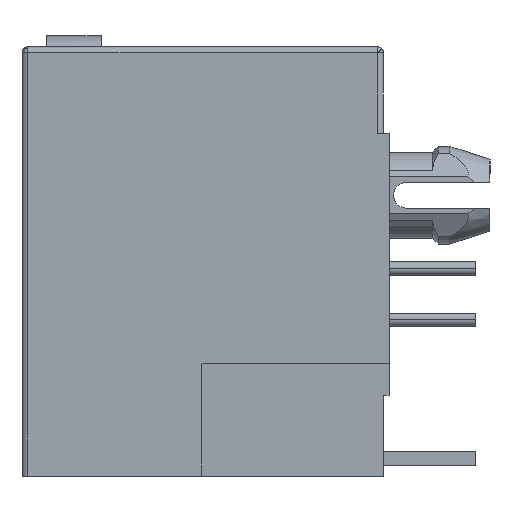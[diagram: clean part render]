
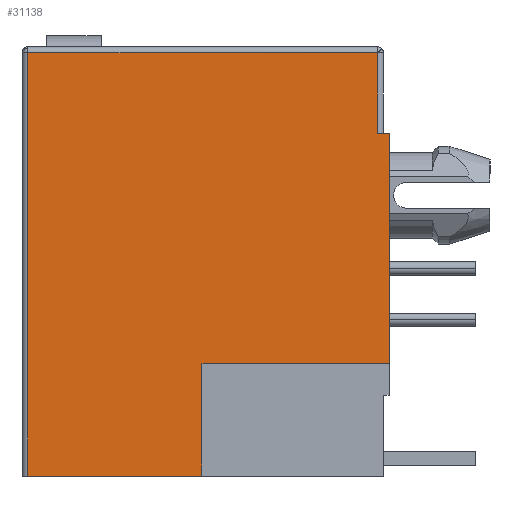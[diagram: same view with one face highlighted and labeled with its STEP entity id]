
A CAD part, left-side view. The second image highlights one B-rep face of the part: STEP entity #31138.
In plain terms, the highlighted planar face has unit normal (-1, 0, 0).
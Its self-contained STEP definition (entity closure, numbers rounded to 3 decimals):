
#608 = AXIS2_PLACEMENT_3D ( 'NONE', #10831, #44853, #58701 ) ;
#704 = CARTESIAN_POINT ( 'NONE',  ( -8.025, -0.125, -3.475 ) ) ;
#1014 = DIRECTION ( 'NONE',  ( 0., 0., 1. ) ) ;
#3329 = VECTOR ( 'NONE', #15140, 1000. ) ;
#4079 = LINE ( 'NONE', #29291, #36528 ) ;
#4708 = EDGE_CURVE ( 'NONE', #26105, #23513, #4079, .T. ) ;
#5362 = EDGE_CURVE ( 'NONE', #15642, #38719, #58306, .T. ) ;
#6454 = CARTESIAN_POINT ( 'NONE',  ( -8.025, 0., -7.375 ) ) ;
#9864 = CARTESIAN_POINT ( 'NONE',  ( -8.025, -6.225, 4.525 ) ) ;
#9989 = VECTOR ( 'NONE', #34020, 1000. ) ;
#10191 = EDGE_LOOP ( 'NONE', ( #31812, #27257, #27498, #35029, #23617, #24989, #46596, #56977 ) ) ;
#10323 = CARTESIAN_POINT ( 'NONE',  ( -8.025, 5.925, 26.949 ) ) ;
#10831 = CARTESIAN_POINT ( 'NONE',  ( -8.025, 0., 0. ) ) ;
#11187 = EDGE_CURVE ( 'NONE', #23513, #20671, #41439, .T. ) ;
#12280 = VERTEX_POINT ( 'NONE', #40879 ) ;
#13189 = CARTESIAN_POINT ( 'NONE',  ( -8.025, -6.625, 4.525 ) ) ;
#15140 = DIRECTION ( 'NONE',  ( 0., -1., 0. ) ) ;
#15278 = PLANE ( 'NONE',  #608 ) ;
#15302 = CARTESIAN_POINT ( 'NONE',  ( -8.025, 0., -3.475 ) ) ;
#15557 = VERTEX_POINT ( 'NONE', #38076 ) ;
#15642 = VERTEX_POINT ( 'NONE', #704 ) ;
#20671 = VERTEX_POINT ( 'NONE', #45750 ) ;
#20880 = VECTOR ( 'NONE', #41548, 1000. ) ;
#22451 = CARTESIAN_POINT ( 'NONE',  ( -8.025, 0., 7.325 ) ) ;
#23513 = VERTEX_POINT ( 'NONE', #59737 ) ;
#23617 = ORIENTED_EDGE ( 'NONE', *, *, #4708, .T. ) ;
#24989 = ORIENTED_EDGE ( 'NONE', *, *, #11187, .T. ) ;
#25247 = LINE ( 'NONE', #6454, #3329 ) ;
#25797 = EDGE_CURVE ( 'NONE', #38719, #28147, #35247, .T. ) ;
#26105 = VERTEX_POINT ( 'NONE', #9864 ) ;
#26622 = FACE_OUTER_BOUND ( 'NONE', #10191, .T. ) ;
#27257 = ORIENTED_EDGE ( 'NONE', *, *, #5362, .T. ) ;
#27498 = ORIENTED_EDGE ( 'NONE', *, *, #25797, .T. ) ;
#28147 = VERTEX_POINT ( 'NONE', #13189 ) ;
#29291 = CARTESIAN_POINT ( 'NONE',  ( -8.025, -6.225, 0. ) ) ;
#29880 = VECTOR ( 'NONE', #36576, 1000. ) ;
#31138 = ADVANCED_FACE ( 'NONE', ( #26622 ), #15278, .T. ) ;
#31812 = ORIENTED_EDGE ( 'NONE', *, *, #43399, .T. ) ;
#32151 = DIRECTION ( 'NONE',  ( 0., 1., 0. ) ) ;
#33746 = DIRECTION ( 'NONE',  ( 0., 0., 1. ) ) ;
#34020 = DIRECTION ( 'NONE',  ( 0., 1., 0. ) ) ;
#35029 = ORIENTED_EDGE ( 'NONE', *, *, #61940, .T. ) ;
#35247 = LINE ( 'NONE', #37299, #20880 ) ;
#36528 = VECTOR ( 'NONE', #1014, 1000. ) ;
#36576 = DIRECTION ( 'NONE',  ( 0., 0., 1. ) ) ;
#37299 = CARTESIAN_POINT ( 'NONE',  ( -8.025, -6.625, 0. ) ) ;
#37841 = EDGE_CURVE ( 'NONE', #12280, #20671, #61949, .T. ) ;
#38076 = CARTESIAN_POINT ( 'NONE',  ( -8.025, -0.125, -7.375 ) ) ;
#38719 = VERTEX_POINT ( 'NONE', #55343 ) ;
#39294 = CARTESIAN_POINT ( 'NONE',  ( -8.025, -6.635, 4.525 ) ) ;
#40879 = CARTESIAN_POINT ( 'NONE',  ( -8.025, 5.925, -7.375 ) ) ;
#41439 = LINE ( 'NONE', #22451, #47510 ) ;
#41548 = DIRECTION ( 'NONE',  ( 0., 0., 1. ) ) ;
#43399 = EDGE_CURVE ( 'NONE', #15557, #15642, #48791, .T. ) ;
#44853 = DIRECTION ( 'NONE',  ( -1., 0., 0. ) ) ;
#45750 = CARTESIAN_POINT ( 'NONE',  ( -8.025, 5.925, 7.325 ) ) ;
#46326 = CARTESIAN_POINT ( 'NONE',  ( -8.025, -0.125, 0. ) ) ;
#46596 = ORIENTED_EDGE ( 'NONE', *, *, #37841, .F. ) ;
#47510 = VECTOR ( 'NONE', #32151, 1000. ) ;
#48791 = LINE ( 'NONE', #46326, #29880 ) ;
#51148 = EDGE_CURVE ( 'NONE', #12280, #15557, #25247, .T. ) ;
#55343 = CARTESIAN_POINT ( 'NONE',  ( -8.025, -6.625, -3.475 ) ) ;
#56977 = ORIENTED_EDGE ( 'NONE', *, *, #51148, .T. ) ;
#58306 = LINE ( 'NONE', #15302, #62052 ) ;
#58701 = DIRECTION ( 'NONE',  ( 0., -1., 0. ) ) ;
#58725 = DIRECTION ( 'NONE',  ( 0., -1., 0. ) ) ;
#59737 = CARTESIAN_POINT ( 'NONE',  ( -8.025, -6.225, 7.325 ) ) ;
#60436 = LINE ( 'NONE', #39294, #9989 ) ;
#60444 = VECTOR ( 'NONE', #33746, 1000. ) ;
#61940 = EDGE_CURVE ( 'NONE', #28147, #26105, #60436, .T. ) ;
#61949 = LINE ( 'NONE', #10323, #60444 ) ;
#62052 = VECTOR ( 'NONE', #58725, 1000. ) ;
